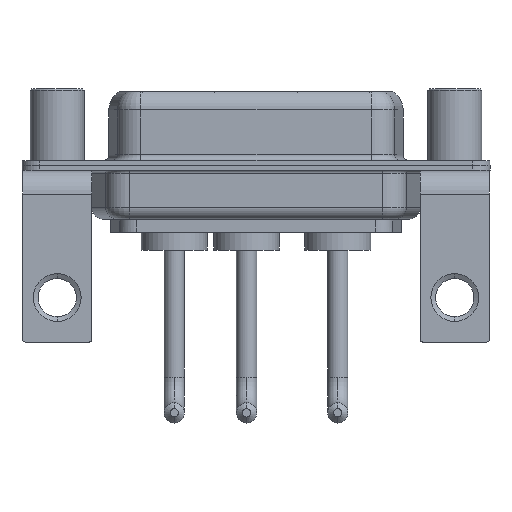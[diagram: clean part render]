
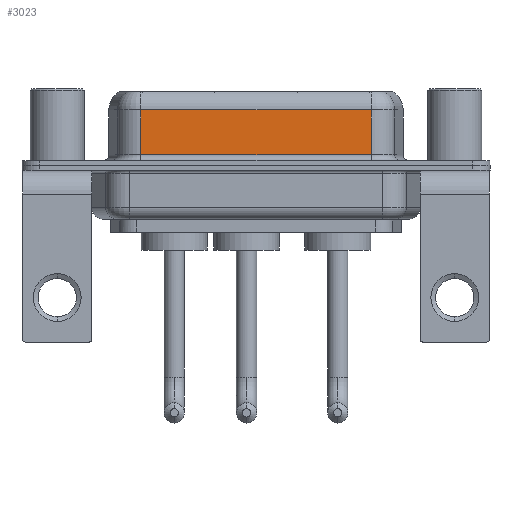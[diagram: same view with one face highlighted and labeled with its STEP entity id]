
A CAD part, front view. The second image highlights one B-rep face of the part: STEP entity #3023.
In plain terms, the highlighted planar face has unit normal (0, -1, 0).
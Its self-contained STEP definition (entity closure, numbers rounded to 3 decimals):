
#20 = CARTESIAN_POINT ( 'NONE',  ( 26.287, -3.95, 0.9 ) ) ;
#310 = CARTESIAN_POINT ( 'NONE',  ( 26.287, -3.95, 6.4 ) ) ;
#505 = DIRECTION ( 'NONE',  ( 0., 0., -1. ) ) ;
#525 = EDGE_LOOP ( 'NONE', ( #3330, #7728, #8232, #7991 ) ) ;
#1739 = DIRECTION ( 'NONE',  ( -1., 0., 0. ) ) ;
#1995 = CARTESIAN_POINT ( 'NONE',  ( 7.013, -3.95, 6.4 ) ) ;
#2154 = DIRECTION ( 'NONE',  ( 0., 0., 1. ) ) ;
#2775 = EDGE_CURVE ( 'NONE', #9591, #4732, #4300, .T. ) ;
#3023 = ADVANCED_FACE ( 'NONE', ( #7093 ), #10892, .F. ) ;
#3330 = ORIENTED_EDGE ( 'NONE', *, *, #10216, .F. ) ;
#3442 = VECTOR ( 'NONE', #1739, 1000. ) ;
#3479 = CARTESIAN_POINT ( 'NONE',  ( 26.287, -3.95, 6.4 ) ) ;
#4300 = LINE ( 'NONE', #6853, #3442 ) ;
#4389 = LINE ( 'NONE', #1995, #15133 ) ;
#4732 = VERTEX_POINT ( 'NONE', #13359 ) ;
#4840 = VECTOR ( 'NONE', #15325, 1000. ) ;
#5840 = DIRECTION ( 'NONE',  ( 0., 0., -1. ) ) ;
#6591 = EDGE_CURVE ( 'NONE', #15807, #9492, #10114, .T. ) ;
#6853 = CARTESIAN_POINT ( 'NONE',  ( 26.287, -3.95, 4.65 ) ) ;
#7093 = FACE_OUTER_BOUND ( 'NONE', #525, .T. ) ;
#7476 = EDGE_CURVE ( 'NONE', #4732, #15807, #4389, .T. ) ;
#7728 = ORIENTED_EDGE ( 'NONE', *, *, #2775, .T. ) ;
#7991 = ORIENTED_EDGE ( 'NONE', *, *, #6591, .T. ) ;
#8232 = ORIENTED_EDGE ( 'NONE', *, *, #7476, .T. ) ;
#8419 = DIRECTION ( 'NONE',  ( 0., 1., 0. ) ) ;
#9459 = CARTESIAN_POINT ( 'NONE',  ( 26.287, -3.95, 4.65 ) ) ;
#9492 = VERTEX_POINT ( 'NONE', #20 ) ;
#9591 = VERTEX_POINT ( 'NONE', #9459 ) ;
#10114 = LINE ( 'NONE', #14009, #4840 ) ;
#10144 = VECTOR ( 'NONE', #5840, 1000. ) ;
#10216 = EDGE_CURVE ( 'NONE', #9591, #9492, #11626, .T. ) ;
#10892 = PLANE ( 'NONE',  #10910 ) ;
#10910 = AXIS2_PLACEMENT_3D ( 'NONE', #3479, #8419, #2154 ) ;
#11626 = LINE ( 'NONE', #310, #10144 ) ;
#12058 = CARTESIAN_POINT ( 'NONE',  ( 7.013, -3.95, 0.9 ) ) ;
#13359 = CARTESIAN_POINT ( 'NONE',  ( 7.013, -3.95, 4.65 ) ) ;
#14009 = CARTESIAN_POINT ( 'NONE',  ( 26.287, -3.95, 0.9 ) ) ;
#15133 = VECTOR ( 'NONE', #505, 1000. ) ;
#15325 = DIRECTION ( 'NONE',  ( 1., 0., 0. ) ) ;
#15807 = VERTEX_POINT ( 'NONE', #12058 ) ;
